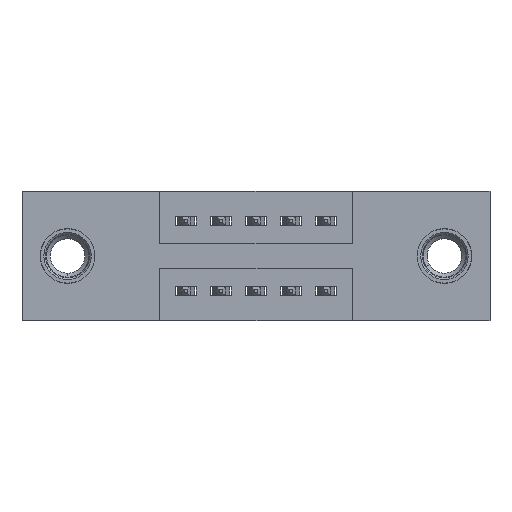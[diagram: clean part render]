
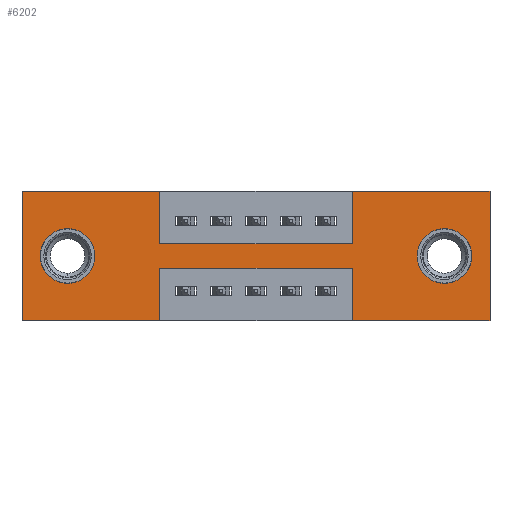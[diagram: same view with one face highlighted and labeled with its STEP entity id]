
A CAD part, front view. The second image highlights one B-rep face of the part: STEP entity #6202.
In plain terms, the highlighted planar face has unit normal (0, -1, 0).
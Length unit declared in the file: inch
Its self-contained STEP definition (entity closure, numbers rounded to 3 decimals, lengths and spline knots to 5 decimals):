
#209 = DIRECTION ( 'NONE',  ( -1., 0., 0. ) ) ;
#287 = CIRCLE ( 'NONE', #3430, 0.078 ) ;
#342 = CARTESIAN_POINT ( 'NONE',  ( 0.9425, 0., -0.37 ) ) ;
#570 = LINE ( 'NONE', #6911, #826 ) ;
#582 = VECTOR ( 'NONE', #3384, 39.37008 ) ;
#702 = VECTOR ( 'NONE', #10112, 39.37008 ) ;
#785 = VECTOR ( 'NONE', #8632, 39.37008 ) ;
#826 = VECTOR ( 'NONE', #1413, 39.37008 ) ;
#927 = CARTESIAN_POINT ( 'NONE',  ( 0.3925, 0., 0. ) ) ;
#973 = CARTESIAN_POINT ( 'NONE',  ( 1.335, 0., 0. ) ) ;
#1164 = EDGE_CURVE ( 'NONE', #1558, #2891, #10120, .T. ) ;
#1218 = DIRECTION ( 'NONE',  ( 0., 1., 0. ) ) ;
#1266 = VECTOR ( 'NONE', #8516, 39.37008 ) ;
#1275 = CARTESIAN_POINT ( 'NONE',  ( 0.13, 0., -0.263 ) ) ;
#1324 = VERTEX_POINT ( 'NONE', #4126 ) ;
#1331 = EDGE_CURVE ( 'NONE', #9489, #1324, #4955, .T. ) ;
#1392 = LINE ( 'NONE', #5406, #785 ) ;
#1413 = DIRECTION ( 'NONE',  ( 1., 0., 0. ) ) ;
#1439 = CARTESIAN_POINT ( 'NONE',  ( 0.9425, 0., -0.22 ) ) ;
#1545 = ORIENTED_EDGE ( 'NONE', *, *, #8034, .T. ) ;
#1558 = VERTEX_POINT ( 'NONE', #1275 ) ;
#1635 = VERTEX_POINT ( 'NONE', #7743 ) ;
#1676 = EDGE_CURVE ( 'NONE', #7233, #9489, #570, .T. ) ;
#1711 = AXIS2_PLACEMENT_3D ( 'NONE', #2792, #9079, #5950 ) ;
#1717 = LINE ( 'NONE', #9397, #6321 ) ;
#1861 = FACE_BOUND ( 'NONE', #3626, .T. ) ;
#1885 = EDGE_CURVE ( 'NONE', #2002, #6269, #9477, .T. ) ;
#2002 = VERTEX_POINT ( 'NONE', #7358 ) ;
#2023 = LINE ( 'NONE', #5084, #5532 ) ;
#2029 = DIRECTION ( 'NONE',  ( 0., 0., -1. ) ) ;
#2130 = VERTEX_POINT ( 'NONE', #3683 ) ;
#2200 = CIRCLE ( 'NONE', #9951, 0.078 ) ;
#2421 = CARTESIAN_POINT ( 'NONE',  ( 0., 0., 0. ) ) ;
#2422 = AXIS2_PLACEMENT_3D ( 'NONE', #3141, #8344, #3932 ) ;
#2467 = EDGE_CURVE ( 'NONE', #1324, #2002, #3471, .T. ) ;
#2498 = VERTEX_POINT ( 'NONE', #927 ) ;
#2540 = LINE ( 'NONE', #2421, #3249 ) ;
#2674 = EDGE_LOOP ( 'NONE', ( #9958, #7444, #9350, #8594, #4013, #5003, #7947, #4589, #9422, #3974, #7526, #6406 ) ) ;
#2724 = EDGE_CURVE ( 'NONE', #8640, #8603, #6893, .T. ) ;
#2781 = CARTESIAN_POINT ( 'NONE',  ( 1.205, 0., -0.185 ) ) ;
#2792 = CARTESIAN_POINT ( 'NONE',  ( 0., 0., -0.37 ) ) ;
#2806 = VERTEX_POINT ( 'NONE', #5168 ) ;
#2891 = VERTEX_POINT ( 'NONE', #7524 ) ;
#3061 = CARTESIAN_POINT ( 'NONE',  ( 0., 0., 0. ) ) ;
#3078 = CARTESIAN_POINT ( 'NONE',  ( 0.3925, 0., -0.37 ) ) ;
#3086 = CIRCLE ( 'NONE', #3895, 0.078 ) ;
#3141 = CARTESIAN_POINT ( 'NONE',  ( 0.13, 0., -0.185 ) ) ;
#3217 = CARTESIAN_POINT ( 'NONE',  ( 1.205, 0., -0.107 ) ) ;
#3249 = VECTOR ( 'NONE', #7858, 39.37008 ) ;
#3377 = CARTESIAN_POINT ( 'NONE',  ( 0.3925, 0., 0. ) ) ;
#3384 = DIRECTION ( 'NONE',  ( 0., 0., -1. ) ) ;
#3430 = AXIS2_PLACEMENT_3D ( 'NONE', #2781, #5166, #2029 ) ;
#3471 = LINE ( 'NONE', #7883, #6379 ) ;
#3546 = CARTESIAN_POINT ( 'NONE',  ( 1.205, 0., -0.185 ) ) ;
#3626 = EDGE_LOOP ( 'NONE', ( #5789, #8665 ) ) ;
#3683 = CARTESIAN_POINT ( 'NONE',  ( 0., 0., -0.37 ) ) ;
#3782 = DIRECTION ( 'NONE',  ( 0., 1., 0. ) ) ;
#3810 = EDGE_CURVE ( 'NONE', #6449, #4143, #287, .T. ) ;
#3846 = LINE ( 'NONE', #3078, #702 ) ;
#3895 = AXIS2_PLACEMENT_3D ( 'NONE', #6881, #3782, #5989 ) ;
#3932 = DIRECTION ( 'NONE',  ( 0., 0., 1. ) ) ;
#3957 = DIRECTION ( 'NONE',  ( 1., 0., 0. ) ) ;
#3974 = ORIENTED_EDGE ( 'NONE', *, *, #4727, .F. ) ;
#4013 = ORIENTED_EDGE ( 'NONE', *, *, #1885, .F. ) ;
#4059 = EDGE_CURVE ( 'NONE', #2130, #5241, #1392, .T. ) ;
#4126 = CARTESIAN_POINT ( 'NONE',  ( 0.9425, 0., 0. ) ) ;
#4143 = VERTEX_POINT ( 'NONE', #3217 ) ;
#4589 = ORIENTED_EDGE ( 'NONE', *, *, #1676, .F. ) ;
#4727 = EDGE_CURVE ( 'NONE', #5241, #2498, #2540, .T. ) ;
#4955 = LINE ( 'NONE', #9548, #6045 ) ;
#4965 = CARTESIAN_POINT ( 'NONE',  ( 1.335, 0., -0.37 ) ) ;
#5003 = ORIENTED_EDGE ( 'NONE', *, *, #2467, .F. ) ;
#5006 = EDGE_CURVE ( 'NONE', #8603, #2806, #2023, .T. ) ;
#5084 = CARTESIAN_POINT ( 'NONE',  ( 0.3925, 0., -0.22 ) ) ;
#5166 = DIRECTION ( 'NONE',  ( 0., 1., 0. ) ) ;
#5168 = CARTESIAN_POINT ( 'NONE',  ( 0.3925, 0., -0.22 ) ) ;
#5181 = DIRECTION ( 'NONE',  ( -1., 0., 0. ) ) ;
#5185 = EDGE_CURVE ( 'NONE', #2891, #1558, #3086, .T. ) ;
#5241 = VERTEX_POINT ( 'NONE', #3061 ) ;
#5288 = CARTESIAN_POINT ( 'NONE',  ( 0., 0., -0.37 ) ) ;
#5406 = CARTESIAN_POINT ( 'NONE',  ( 0., 0., 0. ) ) ;
#5524 = EDGE_CURVE ( 'NONE', #6269, #8640, #9818, .T. ) ;
#5532 = VECTOR ( 'NONE', #5181, 39.37008 ) ;
#5789 = ORIENTED_EDGE ( 'NONE', *, *, #5185, .T. ) ;
#5950 = DIRECTION ( 'NONE',  ( 0., 0., -1. ) ) ;
#5977 = CARTESIAN_POINT ( 'NONE',  ( 1.205, 0., -0.263 ) ) ;
#5989 = DIRECTION ( 'NONE',  ( 0., 0., 1. ) ) ;
#6045 = VECTOR ( 'NONE', #6466, 39.37008 ) ;
#6091 = CARTESIAN_POINT ( 'NONE',  ( 0.3925, 0., -0.15 ) ) ;
#6202 = ADVANCED_FACE ( 'NONE', ( #6593, #1861, #8444 ), #9913, .T. ) ;
#6269 = VERTEX_POINT ( 'NONE', #4965 ) ;
#6321 = VECTOR ( 'NONE', #209, 39.37008 ) ;
#6379 = VECTOR ( 'NONE', #3957, 39.37008 ) ;
#6406 = ORIENTED_EDGE ( 'NONE', *, *, #7518, .F. ) ;
#6449 = VERTEX_POINT ( 'NONE', #5977 ) ;
#6466 = DIRECTION ( 'NONE',  ( 0., 0., 1. ) ) ;
#6593 = FACE_BOUND ( 'NONE', #9546, .T. ) ;
#6785 = CARTESIAN_POINT ( 'NONE',  ( 0.9425, 0., -0.15 ) ) ;
#6881 = CARTESIAN_POINT ( 'NONE',  ( 0.13, 0., -0.185 ) ) ;
#6893 = LINE ( 'NONE', #342, #8375 ) ;
#6911 = CARTESIAN_POINT ( 'NONE',  ( 0.3925, 0., -0.15 ) ) ;
#7196 = DIRECTION ( 'NONE',  ( 0., 0., -1. ) ) ;
#7233 = VERTEX_POINT ( 'NONE', #6091 ) ;
#7358 = CARTESIAN_POINT ( 'NONE',  ( 1.335, 0., 0. ) ) ;
#7444 = ORIENTED_EDGE ( 'NONE', *, *, #5006, .F. ) ;
#7518 = EDGE_CURVE ( 'NONE', #1635, #2130, #1717, .T. ) ;
#7524 = CARTESIAN_POINT ( 'NONE',  ( 0.13, 0., -0.107 ) ) ;
#7526 = ORIENTED_EDGE ( 'NONE', *, *, #4059, .F. ) ;
#7743 = CARTESIAN_POINT ( 'NONE',  ( 0.3925, 0., -0.37 ) ) ;
#7858 = DIRECTION ( 'NONE',  ( 1., 0., 0. ) ) ;
#7883 = CARTESIAN_POINT ( 'NONE',  ( 0., 0., 0. ) ) ;
#7947 = ORIENTED_EDGE ( 'NONE', *, *, #1331, .F. ) ;
#8034 = EDGE_CURVE ( 'NONE', #4143, #6449, #2200, .T. ) ;
#8155 = DIRECTION ( 'NONE',  ( 0., 0., 1. ) ) ;
#8344 = DIRECTION ( 'NONE',  ( 0., 1., 0. ) ) ;
#8375 = VECTOR ( 'NONE', #8155, 39.37008 ) ;
#8444 = FACE_OUTER_BOUND ( 'NONE', #2674, .T. ) ;
#8505 = ORIENTED_EDGE ( 'NONE', *, *, #3810, .T. ) ;
#8516 = DIRECTION ( 'NONE',  ( -1., 0., 0. ) ) ;
#8552 = EDGE_CURVE ( 'NONE', #2498, #7233, #9123, .T. ) ;
#8594 = ORIENTED_EDGE ( 'NONE', *, *, #5524, .F. ) ;
#8603 = VERTEX_POINT ( 'NONE', #1439 ) ;
#8626 = VECTOR ( 'NONE', #7196, 39.37008 ) ;
#8632 = DIRECTION ( 'NONE',  ( 0., 0., 1. ) ) ;
#8640 = VERTEX_POINT ( 'NONE', #9934 ) ;
#8665 = ORIENTED_EDGE ( 'NONE', *, *, #1164, .T. ) ;
#9022 = DIRECTION ( 'NONE',  ( 0., 0., -1. ) ) ;
#9079 = DIRECTION ( 'NONE',  ( 0., -1., 0. ) ) ;
#9123 = LINE ( 'NONE', #3377, #582 ) ;
#9350 = ORIENTED_EDGE ( 'NONE', *, *, #2724, .F. ) ;
#9397 = CARTESIAN_POINT ( 'NONE',  ( 0., 0., -0.37 ) ) ;
#9422 = ORIENTED_EDGE ( 'NONE', *, *, #8552, .F. ) ;
#9477 = LINE ( 'NONE', #973, #8626 ) ;
#9489 = VERTEX_POINT ( 'NONE', #6785 ) ;
#9546 = EDGE_LOOP ( 'NONE', ( #1545, #8505 ) ) ;
#9548 = CARTESIAN_POINT ( 'NONE',  ( 0.9425, 0., 0. ) ) ;
#9818 = LINE ( 'NONE', #5288, #1266 ) ;
#9913 = PLANE ( 'NONE',  #1711 ) ;
#9934 = CARTESIAN_POINT ( 'NONE',  ( 0.9425, 0., -0.37 ) ) ;
#9951 = AXIS2_PLACEMENT_3D ( 'NONE', #3546, #1218, #9022 ) ;
#9958 = ORIENTED_EDGE ( 'NONE', *, *, #9995, .F. ) ;
#9995 = EDGE_CURVE ( 'NONE', #2806, #1635, #3846, .T. ) ;
#10112 = DIRECTION ( 'NONE',  ( 0., 0., -1. ) ) ;
#10120 = CIRCLE ( 'NONE', #2422, 0.078 ) ;
